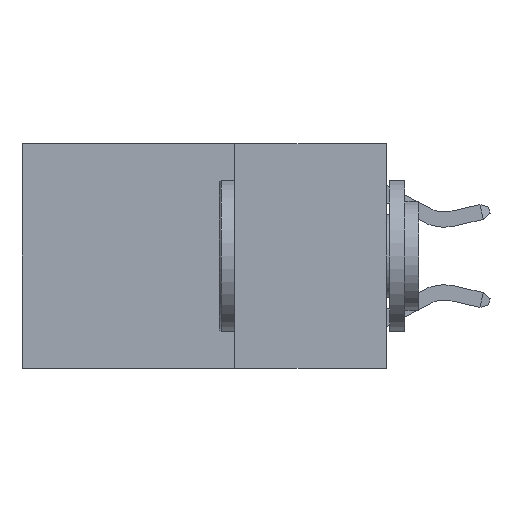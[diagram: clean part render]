
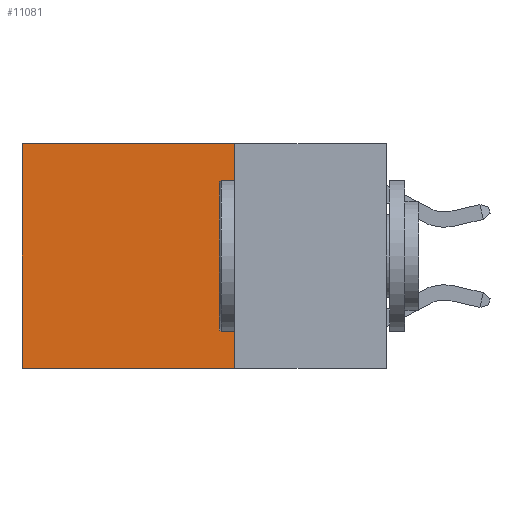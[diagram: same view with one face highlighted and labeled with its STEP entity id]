
A CAD part, left-side view. The second image highlights one B-rep face of the part: STEP entity #11081.
In plain terms, the highlighted planar face has unit normal (-1, 0, 0).
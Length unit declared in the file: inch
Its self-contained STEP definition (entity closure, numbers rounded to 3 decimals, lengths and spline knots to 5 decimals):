
#169 = CARTESIAN_POINT ( 'NONE',  ( 0.2625, 0.6, -0.37 ) ) ;
#220 = LINE ( 'NONE', #11396, #2092 ) ;
#910 = CARTESIAN_POINT ( 'NONE',  ( 0.2625, 0.25, -0.37 ) ) ;
#1431 = LINE ( 'NONE', #4822, #5121 ) ;
#1801 = ORIENTED_EDGE ( 'NONE', *, *, #13792, .T. ) ;
#2042 = CARTESIAN_POINT ( 'NONE',  ( 0.2625, 0.6, 0. ) ) ;
#2092 = VECTOR ( 'NONE', #11465, 39.37008 ) ;
#3235 = VERTEX_POINT ( 'NONE', #4545 ) ;
#3253 = DIRECTION ( 'NONE',  ( 0., 1., 0. ) ) ;
#4545 = CARTESIAN_POINT ( 'NONE',  ( 0.2625, 0.6, 0. ) ) ;
#4689 = EDGE_CURVE ( 'NONE', #7131, #11487, #1431, .T. ) ;
#4822 = CARTESIAN_POINT ( 'NONE',  ( 0.2625, 0.25, 0. ) ) ;
#5121 = VECTOR ( 'NONE', #5785, 39.37008 ) ;
#5223 = FACE_OUTER_BOUND ( 'NONE', #11153, .T. ) ;
#5785 = DIRECTION ( 'NONE',  ( 0., 0., -1. ) ) ;
#6568 = DIRECTION ( 'NONE',  ( 0., 0., -1. ) ) ;
#6591 = ORIENTED_EDGE ( 'NONE', *, *, #4689, .F. ) ;
#6831 = ORIENTED_EDGE ( 'NONE', *, *, #10651, .T. ) ;
#7131 = VERTEX_POINT ( 'NONE', #8740 ) ;
#7573 = VECTOR ( 'NONE', #6568, 39.37008 ) ;
#8008 = ORIENTED_EDGE ( 'NONE', *, *, #13687, .F. ) ;
#8740 = CARTESIAN_POINT ( 'NONE',  ( 0.2625, 0.25, 0. ) ) ;
#8803 = DIRECTION ( 'NONE',  ( 1., 0., 0. ) ) ;
#8843 = CARTESIAN_POINT ( 'NONE',  ( 0.2625, 0.25, -0.37 ) ) ;
#9772 = CARTESIAN_POINT ( 'NONE',  ( 0.2625, 0.25, 0. ) ) ;
#10651 = EDGE_CURVE ( 'NONE', #3235, #11139, #12333, .T. ) ;
#10866 = LINE ( 'NONE', #8843, #11121 ) ;
#11081 = ADVANCED_FACE ( 'NONE', ( #5223 ), #13225, .F. ) ;
#11121 = VECTOR ( 'NONE', #3253, 39.37008 ) ;
#11139 = VERTEX_POINT ( 'NONE', #169 ) ;
#11153 = EDGE_LOOP ( 'NONE', ( #6831, #8008, #6591, #1801 ) ) ;
#11331 = AXIS2_PLACEMENT_3D ( 'NONE', #9772, #8803, #14356 ) ;
#11396 = CARTESIAN_POINT ( 'NONE',  ( 0.2625, 0.25, 0. ) ) ;
#11465 = DIRECTION ( 'NONE',  ( 0., 1., 0. ) ) ;
#11487 = VERTEX_POINT ( 'NONE', #910 ) ;
#12333 = LINE ( 'NONE', #2042, #7573 ) ;
#13225 = PLANE ( 'NONE',  #11331 ) ;
#13687 = EDGE_CURVE ( 'NONE', #11487, #11139, #10866, .T. ) ;
#13792 = EDGE_CURVE ( 'NONE', #7131, #3235, #220, .T. ) ;
#14356 = DIRECTION ( 'NONE',  ( 0., 0., -1. ) ) ;
